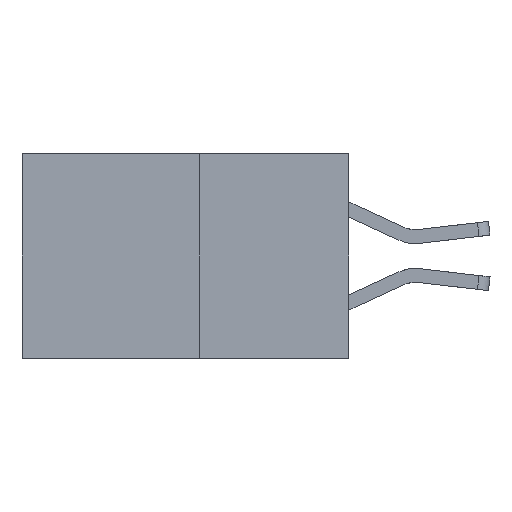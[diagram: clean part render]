
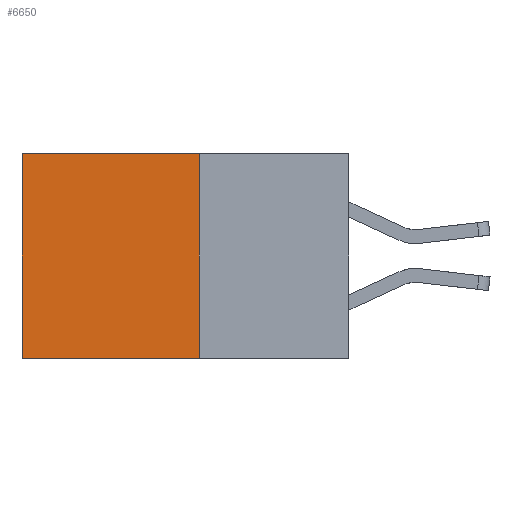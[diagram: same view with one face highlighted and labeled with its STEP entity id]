
A CAD part, left-side view. The second image highlights one B-rep face of the part: STEP entity #6650.
In plain terms, the highlighted planar face has unit normal (-1, 0, 0).
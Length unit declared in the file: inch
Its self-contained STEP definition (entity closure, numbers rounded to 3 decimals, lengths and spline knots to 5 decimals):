
#168 = EDGE_CURVE ( 'NONE', #6461, #6556, #6984, .T. ) ;
#379 = DIRECTION ( 'NONE',  ( 0., 1., 0. ) ) ;
#467 = ORIENTED_EDGE ( 'NONE', *, *, #168, .T. ) ;
#780 = CARTESIAN_POINT ( 'NONE',  ( 0.277, 0.27, -0.37 ) ) ;
#829 = ORIENTED_EDGE ( 'NONE', *, *, #1176, .F. ) ;
#859 = VECTOR ( 'NONE', #4383, 39.37008 ) ;
#981 = EDGE_LOOP ( 'NONE', ( #467, #829, #3795, #7529 ) ) ;
#1041 = EDGE_CURVE ( 'NONE', #5730, #6461, #6108, .T. ) ;
#1176 = EDGE_CURVE ( 'NONE', #4083, #6556, #9204, .T. ) ;
#1370 = AXIS2_PLACEMENT_3D ( 'NONE', #5856, #5704, #5694 ) ;
#1486 = DIRECTION ( 'NONE',  ( 0., 0., -1. ) ) ;
#1607 = EDGE_CURVE ( 'NONE', #5730, #4083, #6432, .T. ) ;
#3653 = CARTESIAN_POINT ( 'NONE',  ( 0.277, 0.27, -0.37 ) ) ;
#3795 = ORIENTED_EDGE ( 'NONE', *, *, #1607, .F. ) ;
#4083 = VERTEX_POINT ( 'NONE', #4328 ) ;
#4205 = CARTESIAN_POINT ( 'NONE',  ( 0.277, 0.59, -0.37 ) ) ;
#4328 = CARTESIAN_POINT ( 'NONE',  ( 0.277, 0.27, -0.37 ) ) ;
#4383 = DIRECTION ( 'NONE',  ( 0., 1., 0. ) ) ;
#4922 = CARTESIAN_POINT ( 'NONE',  ( 0.277, 0.27, 0. ) ) ;
#5694 = DIRECTION ( 'NONE',  ( 0., 0., -1. ) ) ;
#5704 = DIRECTION ( 'NONE',  ( 1., 0., 0. ) ) ;
#5730 = VERTEX_POINT ( 'NONE', #8111 ) ;
#5752 = PLANE ( 'NONE',  #1370 ) ;
#5856 = CARTESIAN_POINT ( 'NONE',  ( 0.277, 0.27, -0.37 ) ) ;
#6108 = LINE ( 'NONE', #4922, #7936 ) ;
#6432 = LINE ( 'NONE', #3653, #10038 ) ;
#6461 = VERTEX_POINT ( 'NONE', #6605 ) ;
#6556 = VERTEX_POINT ( 'NONE', #6560 ) ;
#6560 = CARTESIAN_POINT ( 'NONE',  ( 0.277, 0.59, -0.37 ) ) ;
#6605 = CARTESIAN_POINT ( 'NONE',  ( 0.277, 0.59, 0. ) ) ;
#6650 = ADVANCED_FACE ( 'NONE', ( #9789 ), #5752, .F. ) ;
#6984 = LINE ( 'NONE', #4205, #8520 ) ;
#7529 = ORIENTED_EDGE ( 'NONE', *, *, #1041, .T. ) ;
#7936 = VECTOR ( 'NONE', #379, 39.37008 ) ;
#8111 = CARTESIAN_POINT ( 'NONE',  ( 0.277, 0.27, 0. ) ) ;
#8520 = VECTOR ( 'NONE', #8823, 39.37008 ) ;
#8823 = DIRECTION ( 'NONE',  ( 0., 0., -1. ) ) ;
#9204 = LINE ( 'NONE', #780, #859 ) ;
#9789 = FACE_OUTER_BOUND ( 'NONE', #981, .T. ) ;
#10038 = VECTOR ( 'NONE', #1486, 39.37008 ) ;
